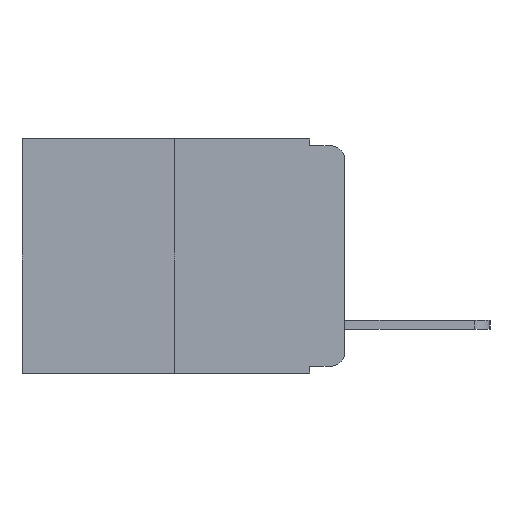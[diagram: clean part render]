
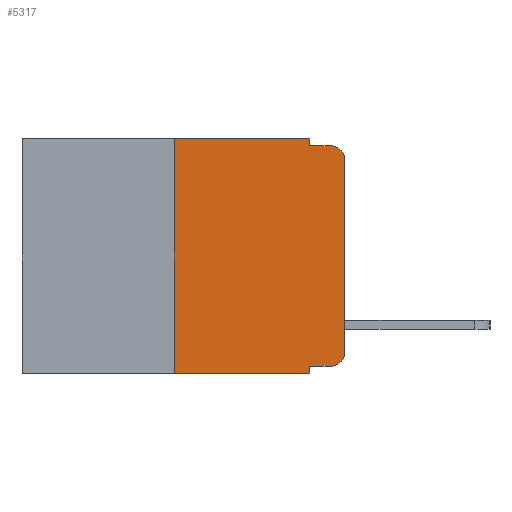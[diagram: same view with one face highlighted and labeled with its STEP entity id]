
A CAD part, left-side view. The second image highlights one B-rep face of the part: STEP entity #5317.
In plain terms, the highlighted planar face has unit normal (-1, 0, 0).
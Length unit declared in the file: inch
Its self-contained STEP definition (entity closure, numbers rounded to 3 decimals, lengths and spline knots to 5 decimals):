
#41 = DIRECTION ( 'NONE',  ( 0., 0., -1. ) ) ;
#246 = ORIENTED_EDGE ( 'NONE', *, *, #7223, .T. ) ;
#596 = EDGE_CURVE ( 'NONE', #6305, #1062, #9998, .T. ) ;
#980 = DIRECTION ( 'NONE',  ( 1., 0., 0. ) ) ;
#1024 = CARTESIAN_POINT ( 'NONE',  ( 0., 0.473, 0. ) ) ;
#1062 = VERTEX_POINT ( 'NONE', #8786 ) ;
#1197 = LINE ( 'NONE', #5198, #8601 ) ;
#1508 = CARTESIAN_POINT ( 'NONE',  ( 0., 0.051, -0.343 ) ) ;
#1615 = AXIS2_PLACEMENT_3D ( 'NONE', #4000, #980, #4780 ) ;
#1670 = CIRCLE ( 'NONE', #12569, 0.02 ) ;
#1917 = EDGE_LOOP ( 'NONE', ( #10639, #8776, #7097, #7192, #10592, #6963, #5057, #5034, #246, #12050 ) ) ;
#2035 = CARTESIAN_POINT ( 'NONE',  ( 0., 0.02, -0.313 ) ) ;
#2068 = CARTESIAN_POINT ( 'NONE',  ( 0., 0.25, 0. ) ) ;
#2878 = EDGE_CURVE ( 'NONE', #12964, #5464, #6151, .T. ) ;
#3186 = CARTESIAN_POINT ( 'NONE',  ( 0., 0.473, -0.343 ) ) ;
#3224 = EDGE_CURVE ( 'NONE', #8252, #7729, #3447, .T. ) ;
#3275 = LINE ( 'NONE', #9144, #5335 ) ;
#3344 = CARTESIAN_POINT ( 'NONE',  ( 0., 0., -0.03 ) ) ;
#3447 = LINE ( 'NONE', #3186, #10629 ) ;
#3551 = VERTEX_POINT ( 'NONE', #4010 ) ;
#3677 = LINE ( 'NONE', #7650, #5502 ) ;
#3935 = DIRECTION ( 'NONE',  ( -1., 0., 0. ) ) ;
#4000 = CARTESIAN_POINT ( 'NONE',  ( 0., 0.473, 0. ) ) ;
#4010 = CARTESIAN_POINT ( 'NONE',  ( 0., 0.02, -0.333 ) ) ;
#4333 = CARTESIAN_POINT ( 'NONE',  ( 0., 0.02, -0.01 ) ) ;
#4436 = CARTESIAN_POINT ( 'NONE',  ( 0., 0., 0. ) ) ;
#4571 = EDGE_CURVE ( 'NONE', #7677, #7729, #3275, .T. ) ;
#4699 = EDGE_CURVE ( 'NONE', #8201, #11985, #6333, .T. ) ;
#4780 = DIRECTION ( 'NONE',  ( 0., 0., -1. ) ) ;
#4979 = VECTOR ( 'NONE', #5041, 39.37008 ) ;
#5034 = ORIENTED_EDGE ( 'NONE', *, *, #4571, .F. ) ;
#5041 = DIRECTION ( 'NONE',  ( 0., -1., 0. ) ) ;
#5057 = ORIENTED_EDGE ( 'NONE', *, *, #3224, .T. ) ;
#5173 = VECTOR ( 'NONE', #9591, 39.37008 ) ;
#5198 = CARTESIAN_POINT ( 'NONE',  ( 0., 0.051, -0.333 ) ) ;
#5317 = ADVANCED_FACE ( 'NONE', ( #7783 ), #5966, .F. ) ;
#5335 = VECTOR ( 'NONE', #41, 39.37008 ) ;
#5464 = VERTEX_POINT ( 'NONE', #4333 ) ;
#5502 = VECTOR ( 'NONE', #8747, 39.37008 ) ;
#5561 = DIRECTION ( 'NONE',  ( 0., 0., -1. ) ) ;
#5809 = CARTESIAN_POINT ( 'NONE',  ( 0., 0.051, 0. ) ) ;
#5915 = VECTOR ( 'NONE', #5561, 39.37008 ) ;
#5966 = PLANE ( 'NONE',  #1615 ) ;
#6151 = LINE ( 'NONE', #9091, #4979 ) ;
#6305 = VERTEX_POINT ( 'NONE', #2068 ) ;
#6333 = LINE ( 'NONE', #4436, #5173 ) ;
#6578 = CARTESIAN_POINT ( 'NONE',  ( 0., 0.25, -0.343 ) ) ;
#6963 = ORIENTED_EDGE ( 'NONE', *, *, #11646, .F. ) ;
#7097 = ORIENTED_EDGE ( 'NONE', *, *, #2878, .F. ) ;
#7192 = ORIENTED_EDGE ( 'NONE', *, *, #9634, .F. ) ;
#7223 = EDGE_CURVE ( 'NONE', #7677, #3551, #1197, .T. ) ;
#7396 = AXIS2_PLACEMENT_3D ( 'NONE', #2035, #3935, #8040 ) ;
#7650 = CARTESIAN_POINT ( 'NONE',  ( 0., 0.25, 0. ) ) ;
#7677 = VERTEX_POINT ( 'NONE', #8103 ) ;
#7682 = DIRECTION ( 'NONE',  ( 0., 0., -1. ) ) ;
#7729 = VERTEX_POINT ( 'NONE', #1508 ) ;
#7760 = LINE ( 'NONE', #5809, #5915 ) ;
#7783 = FACE_OUTER_BOUND ( 'NONE', #1917, .T. ) ;
#8040 = DIRECTION ( 'NONE',  ( 0., 0., -1. ) ) ;
#8103 = CARTESIAN_POINT ( 'NONE',  ( 0., 0.051, -0.333 ) ) ;
#8201 = VERTEX_POINT ( 'NONE', #10508 ) ;
#8252 = VERTEX_POINT ( 'NONE', #6578 ) ;
#8362 = EDGE_CURVE ( 'NONE', #11985, #5464, #1670, .T. ) ;
#8601 = VECTOR ( 'NONE', #12213, 39.37008 ) ;
#8747 = DIRECTION ( 'NONE',  ( 0., 0., 1. ) ) ;
#8776 = ORIENTED_EDGE ( 'NONE', *, *, #8362, .T. ) ;
#8786 = CARTESIAN_POINT ( 'NONE',  ( 0., 0.051, 0. ) ) ;
#8915 = CARTESIAN_POINT ( 'NONE',  ( 0., 0.02, -0.03 ) ) ;
#9091 = CARTESIAN_POINT ( 'NONE',  ( 0., 0.051, -0.01 ) ) ;
#9144 = CARTESIAN_POINT ( 'NONE',  ( 0., 0.051, 0. ) ) ;
#9591 = DIRECTION ( 'NONE',  ( 0., 0., 1. ) ) ;
#9634 = EDGE_CURVE ( 'NONE', #1062, #12964, #7760, .T. ) ;
#9998 = LINE ( 'NONE', #1024, #10950 ) ;
#10508 = CARTESIAN_POINT ( 'NONE',  ( 0., 0., -0.313 ) ) ;
#10592 = ORIENTED_EDGE ( 'NONE', *, *, #596, .F. ) ;
#10629 = VECTOR ( 'NONE', #11289, 39.37008 ) ;
#10639 = ORIENTED_EDGE ( 'NONE', *, *, #4699, .T. ) ;
#10950 = VECTOR ( 'NONE', #11544, 39.37008 ) ;
#11289 = DIRECTION ( 'NONE',  ( 0., -1., 0. ) ) ;
#11347 = CIRCLE ( 'NONE', #7396, 0.02 ) ;
#11401 = EDGE_CURVE ( 'NONE', #3551, #8201, #11347, .T. ) ;
#11544 = DIRECTION ( 'NONE',  ( 0., -1., 0. ) ) ;
#11646 = EDGE_CURVE ( 'NONE', #8252, #6305, #3677, .T. ) ;
#11841 = CARTESIAN_POINT ( 'NONE',  ( 0., 0.051, -0.01 ) ) ;
#11985 = VERTEX_POINT ( 'NONE', #3344 ) ;
#12050 = ORIENTED_EDGE ( 'NONE', *, *, #11401, .T. ) ;
#12213 = DIRECTION ( 'NONE',  ( 0., -1., 0. ) ) ;
#12569 = AXIS2_PLACEMENT_3D ( 'NONE', #8915, #12680, #7682 ) ;
#12680 = DIRECTION ( 'NONE',  ( -1., 0., 0. ) ) ;
#12964 = VERTEX_POINT ( 'NONE', #11841 ) ;
